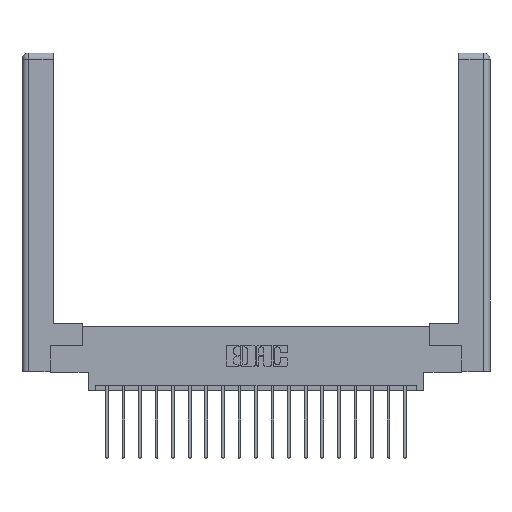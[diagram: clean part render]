
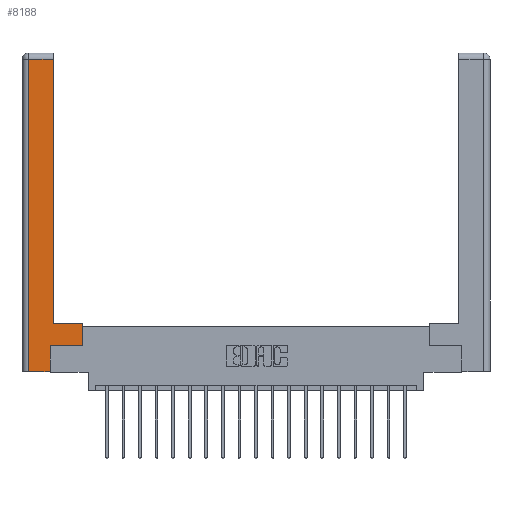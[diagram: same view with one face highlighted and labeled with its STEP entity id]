
A CAD part, top view. The second image highlights one B-rep face of the part: STEP entity #8188.
In plain terms, the highlighted planar face has unit normal (0, 0, 1).
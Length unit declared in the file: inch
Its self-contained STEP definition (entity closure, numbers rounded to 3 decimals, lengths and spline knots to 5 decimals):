
#57 = CARTESIAN_POINT ( 'NONE',  ( 0.265, 0.245, 0. ) ) ;
#71 = CARTESIAN_POINT ( 'NONE',  ( 0., 0., 0. ) ) ;
#147 = VERTEX_POINT ( 'NONE', #7946 ) ;
#472 = EDGE_CURVE ( 'NONE', #4301, #15644, #4631, .T. ) ;
#1096 = ORIENTED_EDGE ( 'NONE', *, *, #10892, .T. ) ;
#1244 = EDGE_CURVE ( 'NONE', #10145, #6680, #12795, .T. ) ;
#1329 = ORIENTED_EDGE ( 'NONE', *, *, #1754, .T. ) ;
#1697 = VECTOR ( 'NONE', #18744, 39.37008 ) ;
#1754 = EDGE_CURVE ( 'NONE', #9142, #4301, #5056, .T. ) ;
#1883 = EDGE_CURVE ( 'NONE', #13879, #9142, #7519, .T. ) ;
#2016 = VERTEX_POINT ( 'NONE', #9255 ) ;
#2074 = ORIENTED_EDGE ( 'NONE', *, *, #8527, .T. ) ;
#2075 = CARTESIAN_POINT ( 'NONE',  ( 0.265, 0., 0. ) ) ;
#3291 = VECTOR ( 'NONE', #10758, 39.37008 ) ;
#3325 = VECTOR ( 'NONE', #16842, 39.37008 ) ;
#3714 = DIRECTION ( 'NONE',  ( -1., 0., 0. ) ) ;
#4301 = VERTEX_POINT ( 'NONE', #57 ) ;
#4631 = LINE ( 'NONE', #10317, #16032 ) ;
#4853 = EDGE_LOOP ( 'NONE', ( #8906, #5085, #2074, #11638, #1329, #11599, #1096, #20273 ) ) ;
#5056 = LINE ( 'NONE', #12908, #16489 ) ;
#5085 = ORIENTED_EDGE ( 'NONE', *, *, #14300, .T. ) ;
#5931 = CARTESIAN_POINT ( 'NONE',  ( 0.0615, 0., 0. ) ) ;
#6511 = LINE ( 'NONE', #16687, #12739 ) ;
#6680 = VERTEX_POINT ( 'NONE', #11756 ) ;
#7519 = LINE ( 'NONE', #14708, #3325 ) ;
#7587 = CARTESIAN_POINT ( 'NONE',  ( 0.0615, 2.94, 0. ) ) ;
#7946 = CARTESIAN_POINT ( 'NONE',  ( 0.565, 0.45, 0. ) ) ;
#8188 = ADVANCED_FACE ( 'NONE', ( #13985 ), #17441, .F. ) ;
#8527 = EDGE_CURVE ( 'NONE', #2016, #13879, #15194, .T. ) ;
#8787 = CARTESIAN_POINT ( 'NONE',  ( 0.295, 3., 0. ) ) ;
#8906 = ORIENTED_EDGE ( 'NONE', *, *, #1244, .T. ) ;
#9142 = VERTEX_POINT ( 'NONE', #2075 ) ;
#9255 = CARTESIAN_POINT ( 'NONE',  ( 0.0615, 2.94, 0. ) ) ;
#9796 = CARTESIAN_POINT ( 'NONE',  ( 0.0615, 0., 0. ) ) ;
#9981 = DIRECTION ( 'NONE',  ( -1., 0., 0. ) ) ;
#10145 = VERTEX_POINT ( 'NONE', #17161 ) ;
#10224 = DIRECTION ( 'NONE',  ( 0., 1., 0. ) ) ;
#10317 = CARTESIAN_POINT ( 'NONE',  ( 0.565, 0.245, 0. ) ) ;
#10758 = DIRECTION ( 'NONE',  ( 0., -1., 0. ) ) ;
#10892 = EDGE_CURVE ( 'NONE', #15644, #147, #6511, .T. ) ;
#11018 = DIRECTION ( 'NONE',  ( 0., 0., -1. ) ) ;
#11599 = ORIENTED_EDGE ( 'NONE', *, *, #472, .T. ) ;
#11638 = ORIENTED_EDGE ( 'NONE', *, *, #1883, .T. ) ;
#11756 = CARTESIAN_POINT ( 'NONE',  ( 0.295, 2.94, 0. ) ) ;
#12739 = VECTOR ( 'NONE', #10224, 39.37008 ) ;
#12795 = LINE ( 'NONE', #8787, #14044 ) ;
#12853 = LINE ( 'NONE', #7587, #1697 ) ;
#12908 = CARTESIAN_POINT ( 'NONE',  ( 0.265, 0.245, 0. ) ) ;
#13233 = CARTESIAN_POINT ( 'NONE',  ( 0.295, 0.45, 0. ) ) ;
#13879 = VERTEX_POINT ( 'NONE', #9796 ) ;
#13985 = FACE_OUTER_BOUND ( 'NONE', #4853, .T. ) ;
#14044 = VECTOR ( 'NONE', #18623, 39.37008 ) ;
#14300 = EDGE_CURVE ( 'NONE', #6680, #2016, #12853, .T. ) ;
#14708 = CARTESIAN_POINT ( 'NONE',  ( 0.265, 0., 0. ) ) ;
#15194 = LINE ( 'NONE', #5931, #3291 ) ;
#15644 = VERTEX_POINT ( 'NONE', #19544 ) ;
#16032 = VECTOR ( 'NONE', #16485, 39.37008 ) ;
#16485 = DIRECTION ( 'NONE',  ( 1., 0., 0. ) ) ;
#16489 = VECTOR ( 'NONE', #19226, 39.37008 ) ;
#16687 = CARTESIAN_POINT ( 'NONE',  ( 0.565, 0.45, 0. ) ) ;
#16842 = DIRECTION ( 'NONE',  ( 1., 0., 0. ) ) ;
#17161 = CARTESIAN_POINT ( 'NONE',  ( 0.295, 0.45, 0. ) ) ;
#17441 = PLANE ( 'NONE',  #18883 ) ;
#18623 = DIRECTION ( 'NONE',  ( 0., 1., 0. ) ) ;
#18744 = DIRECTION ( 'NONE',  ( -1., 0., 0. ) ) ;
#18883 = AXIS2_PLACEMENT_3D ( 'NONE', #71, #11018, #9981 ) ;
#19135 = VECTOR ( 'NONE', #3714, 39.37008 ) ;
#19226 = DIRECTION ( 'NONE',  ( 0., 1., 0. ) ) ;
#19544 = CARTESIAN_POINT ( 'NONE',  ( 0.565, 0.245, 0. ) ) ;
#19776 = EDGE_CURVE ( 'NONE', #147, #10145, #19875, .T. ) ;
#19875 = LINE ( 'NONE', #13233, #19135 ) ;
#20273 = ORIENTED_EDGE ( 'NONE', *, *, #19776, .T. ) ;
